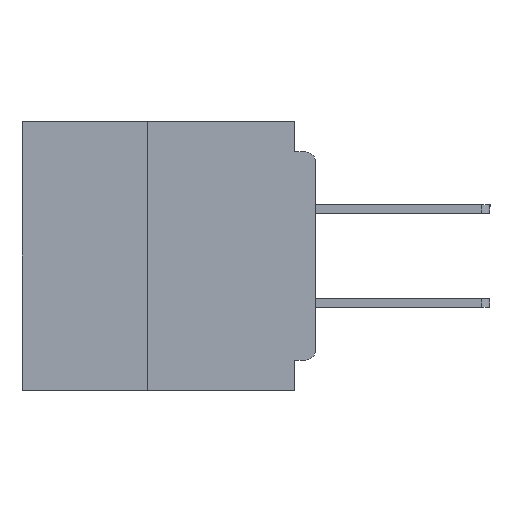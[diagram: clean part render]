
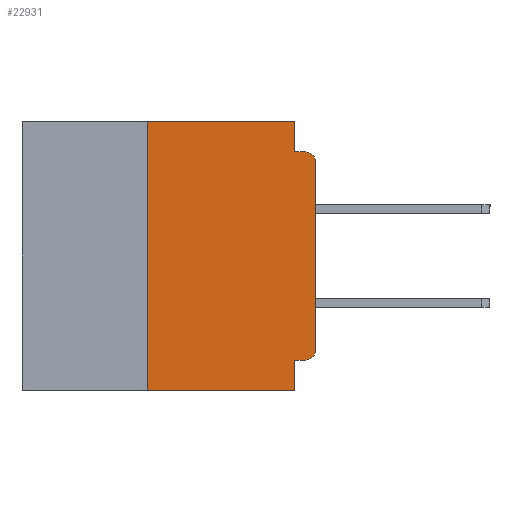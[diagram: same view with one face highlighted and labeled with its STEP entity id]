
A CAD part, left-side view. The second image highlights one B-rep face of the part: STEP entity #22931.
In plain terms, the highlighted planar face has unit normal (-1, 0, 0).
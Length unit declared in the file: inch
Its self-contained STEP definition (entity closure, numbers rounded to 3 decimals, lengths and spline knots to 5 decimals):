
#1302 = CARTESIAN_POINT ( 'NONE',  ( 0., 0.25, -0.4 ) ) ;
#3453 = VERTEX_POINT ( 'NONE', #40714 ) ;
#3769 = VERTEX_POINT ( 'NONE', #23124 ) ;
#4017 = LINE ( 'NONE', #26850, #30515 ) ;
#4049 = ORIENTED_EDGE ( 'NONE', *, *, #40556, .F. ) ;
#4525 = EDGE_CURVE ( 'NONE', #3769, #3453, #4017, .T. ) ;
#4579 = CARTESIAN_POINT ( 'NONE',  ( 0., 0.031, -0.4 ) ) ;
#5369 = EDGE_LOOP ( 'NONE', ( #23748, #19178, #36496, #16740, #54414, #34723, #34847, #24760, #4049, #11261 ) ) ;
#5725 = DIRECTION ( 'NONE',  ( 0., -1., 0. ) ) ;
#6168 = VECTOR ( 'NONE', #8659, 39.37008 ) ;
#7211 = CARTESIAN_POINT ( 'NONE',  ( 0., 0.015, -0.045 ) ) ;
#7493 = CARTESIAN_POINT ( 'NONE',  ( 0., 0.25, 0. ) ) ;
#8239 = CARTESIAN_POINT ( 'NONE',  ( 0., 0., -0.34 ) ) ;
#8408 = CARTESIAN_POINT ( 'NONE',  ( 0., 0.015, -0.355 ) ) ;
#8659 = DIRECTION ( 'NONE',  ( 0., 1., 0. ) ) ;
#8670 = CARTESIAN_POINT ( 'NONE',  ( 0., 0., -0.06 ) ) ;
#8736 = DIRECTION ( 'NONE',  ( 0., 0., -1. ) ) ;
#9989 = FACE_OUTER_BOUND ( 'NONE', #5369, .T. ) ;
#11261 = ORIENTED_EDGE ( 'NONE', *, *, #21579, .T. ) ;
#11537 = DIRECTION ( 'NONE',  ( -1., 0., 0. ) ) ;
#12038 = VERTEX_POINT ( 'NONE', #8670 ) ;
#13100 = VECTOR ( 'NONE', #23687, 39.37008 ) ;
#13862 = DIRECTION ( 'NONE',  ( 0., -1., 0. ) ) ;
#13943 = CARTESIAN_POINT ( 'NONE',  ( 0., 0., -0.355 ) ) ;
#14053 = LINE ( 'NONE', #1302, #29221 ) ;
#15211 = DIRECTION ( 'NONE',  ( 0., 0., -1. ) ) ;
#15598 = AXIS2_PLACEMENT_3D ( 'NONE', #24476, #40384, #8736 ) ;
#16740 = ORIENTED_EDGE ( 'NONE', *, *, #26779, .F. ) ;
#16742 = VECTOR ( 'NONE', #39888, 39.37008 ) ;
#18376 = CARTESIAN_POINT ( 'NONE',  ( 0., 0., 0. ) ) ;
#18569 = CARTESIAN_POINT ( 'NONE',  ( 0., 0.031, -0.355 ) ) ;
#18678 = AXIS2_PLACEMENT_3D ( 'NONE', #29009, #65867, #34265 ) ;
#18990 = CARTESIAN_POINT ( 'NONE',  ( 0., 0., -0.045 ) ) ;
#19118 = EDGE_CURVE ( 'NONE', #31830, #54118, #30819, .T. ) ;
#19160 = PLANE ( 'NONE',  #15598 ) ;
#19178 = ORIENTED_EDGE ( 'NONE', *, *, #36094, .T. ) ;
#19240 = CARTESIAN_POINT ( 'NONE',  ( 0., 0.031, -0.045 ) ) ;
#19991 = CIRCLE ( 'NONE', #45954, 0.015 ) ;
#21579 = EDGE_CURVE ( 'NONE', #21762, #37771, #60275, .T. ) ;
#21762 = VERTEX_POINT ( 'NONE', #8408 ) ;
#22931 = ADVANCED_FACE ( 'NONE', ( #9989 ), #19160, .F. ) ;
#23124 = CARTESIAN_POINT ( 'NONE',  ( 0., 0.25, -0.4 ) ) ;
#23687 = DIRECTION ( 'NONE',  ( 0., 0., 1. ) ) ;
#23748 = ORIENTED_EDGE ( 'NONE', *, *, #44265, .T. ) ;
#24476 = CARTESIAN_POINT ( 'NONE',  ( 0., 0.437, 0. ) ) ;
#24760 = ORIENTED_EDGE ( 'NONE', *, *, #56277, .F. ) ;
#26779 = EDGE_CURVE ( 'NONE', #54118, #51402, #41774, .T. ) ;
#26850 = CARTESIAN_POINT ( 'NONE',  ( 0., 0.437, -0.4 ) ) ;
#27753 = VECTOR ( 'NONE', #63786, 39.37008 ) ;
#29009 = CARTESIAN_POINT ( 'NONE',  ( 0., 0.015, -0.34 ) ) ;
#29221 = VECTOR ( 'NONE', #48956, 39.37008 ) ;
#30515 = VECTOR ( 'NONE', #5725, 39.37008 ) ;
#30819 = LINE ( 'NONE', #55588, #16742 ) ;
#31830 = VERTEX_POINT ( 'NONE', #7493 ) ;
#33972 = VECTOR ( 'NONE', #13862, 39.37008 ) ;
#34265 = DIRECTION ( 'NONE',  ( 0., 0., -1. ) ) ;
#34723 = ORIENTED_EDGE ( 'NONE', *, *, #37565, .F. ) ;
#34847 = ORIENTED_EDGE ( 'NONE', *, *, #4525, .T. ) ;
#36094 = EDGE_CURVE ( 'NONE', #12038, #46521, #19991, .T. ) ;
#36496 = ORIENTED_EDGE ( 'NONE', *, *, #37209, .F. ) ;
#37209 = EDGE_CURVE ( 'NONE', #51402, #46521, #63691, .T. ) ;
#37565 = EDGE_CURVE ( 'NONE', #3769, #31830, #14053, .T. ) ;
#37771 = VERTEX_POINT ( 'NONE', #8239 ) ;
#39888 = DIRECTION ( 'NONE',  ( 0., -1., 0. ) ) ;
#40384 = DIRECTION ( 'NONE',  ( 1., 0., 0. ) ) ;
#40556 = EDGE_CURVE ( 'NONE', #21762, #68058, #51665, .T. ) ;
#40714 = CARTESIAN_POINT ( 'NONE',  ( 0., 0.031, -0.4 ) ) ;
#41774 = LINE ( 'NONE', #42574, #27753 ) ;
#42574 = CARTESIAN_POINT ( 'NONE',  ( 0., 0.031, 0. ) ) ;
#43123 = VECTOR ( 'NONE', #15211, 39.37008 ) ;
#43194 = CARTESIAN_POINT ( 'NONE',  ( 0., 0.015, -0.06 ) ) ;
#44265 = EDGE_CURVE ( 'NONE', #37771, #12038, #65970, .T. ) ;
#45954 = AXIS2_PLACEMENT_3D ( 'NONE', #43194, #11537, #48522 ) ;
#46521 = VERTEX_POINT ( 'NONE', #7211 ) ;
#48522 = DIRECTION ( 'NONE',  ( 0., 0., -1. ) ) ;
#48956 = DIRECTION ( 'NONE',  ( 0., 0., 1. ) ) ;
#51402 = VERTEX_POINT ( 'NONE', #19240 ) ;
#51665 = LINE ( 'NONE', #13943, #6168 ) ;
#54118 = VERTEX_POINT ( 'NONE', #54984 ) ;
#54414 = ORIENTED_EDGE ( 'NONE', *, *, #19118, .F. ) ;
#54984 = CARTESIAN_POINT ( 'NONE',  ( 0., 0.031, 0. ) ) ;
#55588 = CARTESIAN_POINT ( 'NONE',  ( 0., 0.437, 0. ) ) ;
#56277 = EDGE_CURVE ( 'NONE', #68058, #3453, #57184, .T. ) ;
#57184 = LINE ( 'NONE', #4579, #43123 ) ;
#60275 = CIRCLE ( 'NONE', #18678, 0.015 ) ;
#63691 = LINE ( 'NONE', #18990, #33972 ) ;
#63786 = DIRECTION ( 'NONE',  ( 0., 0., -1. ) ) ;
#65867 = DIRECTION ( 'NONE',  ( -1., 0., 0. ) ) ;
#65970 = LINE ( 'NONE', #18376, #13100 ) ;
#68058 = VERTEX_POINT ( 'NONE', #18569 ) ;
